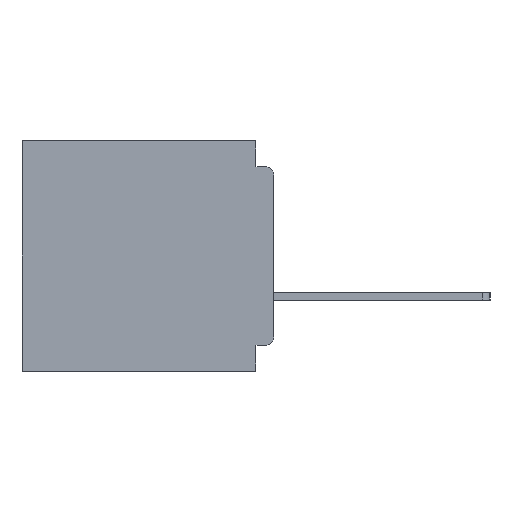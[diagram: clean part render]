
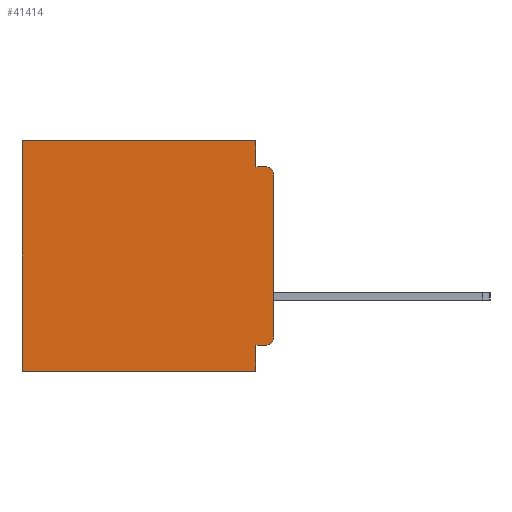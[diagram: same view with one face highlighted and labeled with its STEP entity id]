
A CAD part, left-side view. The second image highlights one B-rep face of the part: STEP entity #41414.
In plain terms, the highlighted planar face has unit normal (-1, 0, 0).
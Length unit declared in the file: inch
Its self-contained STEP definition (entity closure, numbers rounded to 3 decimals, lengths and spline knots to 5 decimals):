
#161 = DIRECTION ( 'NONE',  ( -1., 0., 0. ) ) ;
#304 = CARTESIAN_POINT ( 'NONE',  ( 0.3, 0.031, 0. ) ) ;
#519 = VERTEX_POINT ( 'NONE', #9719 ) ;
#1029 = VERTEX_POINT ( 'NONE', #13330 ) ;
#1396 = ORIENTED_EDGE ( 'NONE', *, *, #23572, .T. ) ;
#1613 = EDGE_CURVE ( 'NONE', #22149, #6372, #40595, .T. ) ;
#1902 = VERTEX_POINT ( 'NONE', #29315 ) ;
#1963 = LINE ( 'NONE', #36731, #36862 ) ;
#2319 = EDGE_CURVE ( 'NONE', #20628, #519, #22244, .T. ) ;
#3703 = DIRECTION ( 'NONE',  ( 1., 0., 0. ) ) ;
#3780 = LINE ( 'NONE', #18183, #37547 ) ;
#3939 = CARTESIAN_POINT ( 'NONE',  ( 0.3, 0.031, -0.4 ) ) ;
#4016 = CARTESIAN_POINT ( 'NONE',  ( 0.3, 0., -0.355 ) ) ;
#4524 = ORIENTED_EDGE ( 'NONE', *, *, #36339, .F. ) ;
#6372 = VERTEX_POINT ( 'NONE', #32271 ) ;
#7363 = CARTESIAN_POINT ( 'NONE',  ( 0.3, 0., -0.06 ) ) ;
#7450 = AXIS2_PLACEMENT_3D ( 'NONE', #10625, #35010, #14131 ) ;
#7749 = EDGE_CURVE ( 'NONE', #24841, #26152, #1963, .T. ) ;
#8841 = CARTESIAN_POINT ( 'NONE',  ( 0.3, 0.437, -0.4 ) ) ;
#9204 = LINE ( 'NONE', #3939, #35933 ) ;
#9719 = CARTESIAN_POINT ( 'NONE',  ( 0.3, 0.437, 0. ) ) ;
#10003 = AXIS2_PLACEMENT_3D ( 'NONE', #17615, #3703, #28106 ) ;
#10625 = CARTESIAN_POINT ( 'NONE',  ( 0.3, 0.015, -0.06 ) ) ;
#11212 = AXIS2_PLACEMENT_3D ( 'NONE', #21144, #161, #24594 ) ;
#11802 = EDGE_CURVE ( 'NONE', #6372, #24648, #9204, .T. ) ;
#12914 = VECTOR ( 'NONE', #25327, 39.37008 ) ;
#13330 = CARTESIAN_POINT ( 'NONE',  ( 0.3, 0.015, -0.045 ) ) ;
#13530 = VECTOR ( 'NONE', #26038, 39.37008 ) ;
#14122 = EDGE_CURVE ( 'NONE', #20628, #1902, #44854, .T. ) ;
#14131 = DIRECTION ( 'NONE',  ( 0., 0., -1. ) ) ;
#15044 = EDGE_CURVE ( 'NONE', #519, #41713, #43033, .T. ) ;
#15300 = ORIENTED_EDGE ( 'NONE', *, *, #14122, .F. ) ;
#15390 = VECTOR ( 'NONE', #21263, 39.37008 ) ;
#17509 = ORIENTED_EDGE ( 'NONE', *, *, #7749, .F. ) ;
#17615 = CARTESIAN_POINT ( 'NONE',  ( 0.3, 0., -0.4 ) ) ;
#17728 = CARTESIAN_POINT ( 'NONE',  ( 0.3, 0.437, -0.4 ) ) ;
#17995 = CARTESIAN_POINT ( 'NONE',  ( 0.3, 0., -0.34 ) ) ;
#18183 = CARTESIAN_POINT ( 'NONE',  ( 0.3, 0., -0.045 ) ) ;
#18251 = FACE_OUTER_BOUND ( 'NONE', #29931, .T. ) ;
#19423 = ORIENTED_EDGE ( 'NONE', *, *, #27360, .F. ) ;
#20628 = VERTEX_POINT ( 'NONE', #304 ) ;
#21144 = CARTESIAN_POINT ( 'NONE',  ( 0.3, 0.015, -0.34 ) ) ;
#21263 = DIRECTION ( 'NONE',  ( 0., 0., -1. ) ) ;
#21992 = ORIENTED_EDGE ( 'NONE', *, *, #15044, .T. ) ;
#22018 = DIRECTION ( 'NONE',  ( 0., 0., -1. ) ) ;
#22149 = VERTEX_POINT ( 'NONE', #37497 ) ;
#22244 = LINE ( 'NONE', #38920, #12914 ) ;
#23572 = EDGE_CURVE ( 'NONE', #22149, #26152, #44982, .T. ) ;
#23826 = DIRECTION ( 'NONE',  ( 0., 1., 0. ) ) ;
#24594 = DIRECTION ( 'NONE',  ( 0., 0., -1. ) ) ;
#24611 = PLANE ( 'NONE',  #10003 ) ;
#24648 = VERTEX_POINT ( 'NONE', #44392 ) ;
#24835 = DIRECTION ( 'NONE',  ( 0., 0., -1. ) ) ;
#24841 = VERTEX_POINT ( 'NONE', #7363 ) ;
#25327 = DIRECTION ( 'NONE',  ( 0., 1., 0. ) ) ;
#26038 = DIRECTION ( 'NONE',  ( 0., 1., 0. ) ) ;
#26152 = VERTEX_POINT ( 'NONE', #17995 ) ;
#27360 = EDGE_CURVE ( 'NONE', #1902, #1029, #3780, .T. ) ;
#27950 = CIRCLE ( 'NONE', #7450, 0.015 ) ;
#28106 = DIRECTION ( 'NONE',  ( 0., 0., -1. ) ) ;
#29315 = CARTESIAN_POINT ( 'NONE',  ( 0.3, 0.031, -0.045 ) ) ;
#29931 = EDGE_LOOP ( 'NONE', ( #17509, #33397, #19423, #15300, #42989, #21992, #4524, #33972, #36717, #1396 ) ) ;
#32271 = CARTESIAN_POINT ( 'NONE',  ( 0.3, 0.031, -0.355 ) ) ;
#33397 = ORIENTED_EDGE ( 'NONE', *, *, #35219, .T. ) ;
#33916 = VECTOR ( 'NONE', #23826, 39.37008 ) ;
#33972 = ORIENTED_EDGE ( 'NONE', *, *, #11802, .F. ) ;
#35010 = DIRECTION ( 'NONE',  ( -1., 0., 0. ) ) ;
#35219 = EDGE_CURVE ( 'NONE', #24841, #1029, #27950, .T. ) ;
#35527 = DIRECTION ( 'NONE',  ( 0., -1., 0. ) ) ;
#35768 = VECTOR ( 'NONE', #22018, 39.37008 ) ;
#35933 = VECTOR ( 'NONE', #24835, 39.37008 ) ;
#36019 = DIRECTION ( 'NONE',  ( 0., 0., -1. ) ) ;
#36339 = EDGE_CURVE ( 'NONE', #24648, #41713, #43012, .T. ) ;
#36717 = ORIENTED_EDGE ( 'NONE', *, *, #1613, .F. ) ;
#36731 = CARTESIAN_POINT ( 'NONE',  ( 0.3, 0., -0.4 ) ) ;
#36862 = VECTOR ( 'NONE', #36019, 39.37008 ) ;
#37497 = CARTESIAN_POINT ( 'NONE',  ( 0.3, 0.015, -0.355 ) ) ;
#37547 = VECTOR ( 'NONE', #35527, 39.37008 ) ;
#38920 = CARTESIAN_POINT ( 'NONE',  ( 0.3, 0., 0. ) ) ;
#40595 = LINE ( 'NONE', #4016, #13530 ) ;
#41414 = ADVANCED_FACE ( 'NONE', ( #18251 ), #24611, .F. ) ;
#41713 = VERTEX_POINT ( 'NONE', #8841 ) ;
#42699 = CARTESIAN_POINT ( 'NONE',  ( 0.3, 0.031, 0. ) ) ;
#42989 = ORIENTED_EDGE ( 'NONE', *, *, #2319, .T. ) ;
#43012 = LINE ( 'NONE', #44308, #33916 ) ;
#43033 = LINE ( 'NONE', #17728, #15390 ) ;
#44308 = CARTESIAN_POINT ( 'NONE',  ( 0.3, 0., -0.4 ) ) ;
#44392 = CARTESIAN_POINT ( 'NONE',  ( 0.3, 0.031, -0.4 ) ) ;
#44854 = LINE ( 'NONE', #42699, #35768 ) ;
#44982 = CIRCLE ( 'NONE', #11212, 0.015 ) ;
